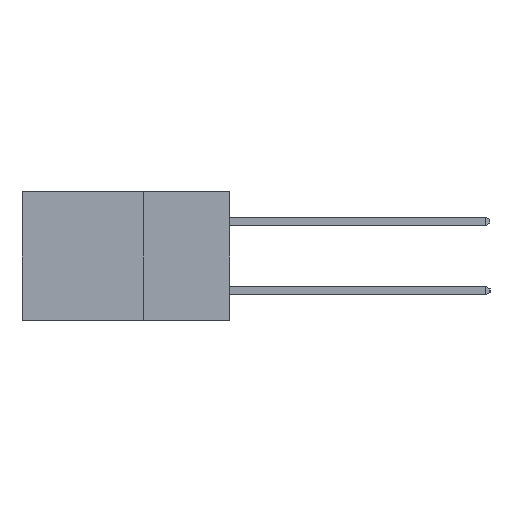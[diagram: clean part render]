
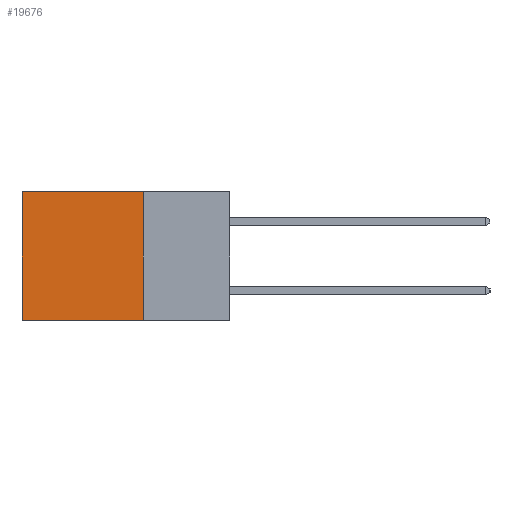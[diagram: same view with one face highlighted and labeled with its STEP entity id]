
A CAD part, left-side view. The second image highlights one B-rep face of the part: STEP entity #19676.
In plain terms, the highlighted planar face has unit normal (-1, 0, 0).
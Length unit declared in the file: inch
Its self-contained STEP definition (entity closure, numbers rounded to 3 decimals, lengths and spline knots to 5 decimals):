
#275 = CARTESIAN_POINT ( 'NONE',  ( 0.2615, 0.6, 0. ) ) ;
#2744 = EDGE_CURVE ( 'NONE', #13418, #18797, #22776, .T. ) ;
#2862 = PLANE ( 'NONE',  #6494 ) ;
#3058 = VECTOR ( 'NONE', #5656, 39.37008 ) ;
#3509 = CARTESIAN_POINT ( 'NONE',  ( 0.2615, 0.25, 0. ) ) ;
#4822 = VERTEX_POINT ( 'NONE', #11522 ) ;
#5656 = DIRECTION ( 'NONE',  ( 0., 0., -1. ) ) ;
#6188 = LINE ( 'NONE', #24183, #6796 ) ;
#6494 = AXIS2_PLACEMENT_3D ( 'NONE', #16304, #18146, #6761 ) ;
#6628 = EDGE_CURVE ( 'NONE', #18797, #18221, #13359, .T. ) ;
#6761 = DIRECTION ( 'NONE',  ( 0., 0., -1. ) ) ;
#6796 = VECTOR ( 'NONE', #15009, 39.37008 ) ;
#7519 = CARTESIAN_POINT ( 'NONE',  ( 0.2615, 0.6, -0.37 ) ) ;
#7699 = DIRECTION ( 'NONE',  ( 0., 0., -1. ) ) ;
#11522 = CARTESIAN_POINT ( 'NONE',  ( 0.2615, 0.25, -0.37 ) ) ;
#11919 = EDGE_CURVE ( 'NONE', #13418, #4822, #19407, .T. ) ;
#12725 = FACE_OUTER_BOUND ( 'NONE', #18528, .T. ) ;
#13359 = LINE ( 'NONE', #7519, #3058 ) ;
#13418 = VERTEX_POINT ( 'NONE', #14211 ) ;
#13489 = CARTESIAN_POINT ( 'NONE',  ( 0.2615, 0.25, -0.37 ) ) ;
#14211 = CARTESIAN_POINT ( 'NONE',  ( 0.2615, 0.25, 0. ) ) ;
#15009 = DIRECTION ( 'NONE',  ( 0., 1., 0. ) ) ;
#15758 = DIRECTION ( 'NONE',  ( 0., 1., 0. ) ) ;
#16304 = CARTESIAN_POINT ( 'NONE',  ( 0.2615, 0.25, -0.37 ) ) ;
#17113 = EDGE_CURVE ( 'NONE', #4822, #18221, #6188, .T. ) ;
#17881 = VECTOR ( 'NONE', #15758, 39.37008 ) ;
#18146 = DIRECTION ( 'NONE',  ( 1., 0., 0. ) ) ;
#18221 = VERTEX_POINT ( 'NONE', #19825 ) ;
#18235 = VECTOR ( 'NONE', #7699, 39.37008 ) ;
#18528 = EDGE_LOOP ( 'NONE', ( #20034, #19980, #20927, #19246 ) ) ;
#18797 = VERTEX_POINT ( 'NONE', #275 ) ;
#19246 = ORIENTED_EDGE ( 'NONE', *, *, #2744, .T. ) ;
#19407 = LINE ( 'NONE', #13489, #18235 ) ;
#19676 = ADVANCED_FACE ( 'NONE', ( #12725 ), #2862, .F. ) ;
#19825 = CARTESIAN_POINT ( 'NONE',  ( 0.2615, 0.6, -0.37 ) ) ;
#19980 = ORIENTED_EDGE ( 'NONE', *, *, #17113, .F. ) ;
#20034 = ORIENTED_EDGE ( 'NONE', *, *, #6628, .T. ) ;
#20927 = ORIENTED_EDGE ( 'NONE', *, *, #11919, .F. ) ;
#22776 = LINE ( 'NONE', #3509, #17881 ) ;
#24183 = CARTESIAN_POINT ( 'NONE',  ( 0.2615, 0.25, -0.37 ) ) ;
